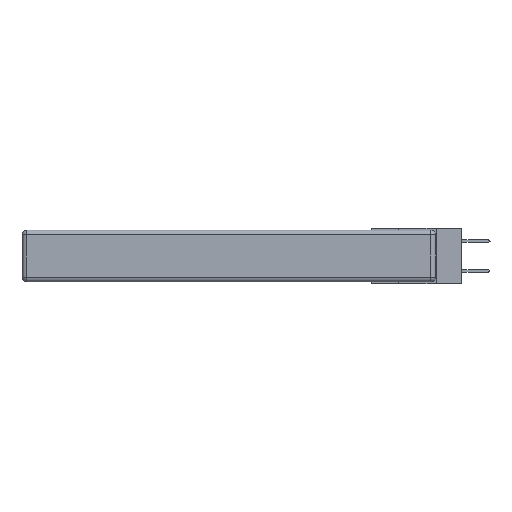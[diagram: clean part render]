
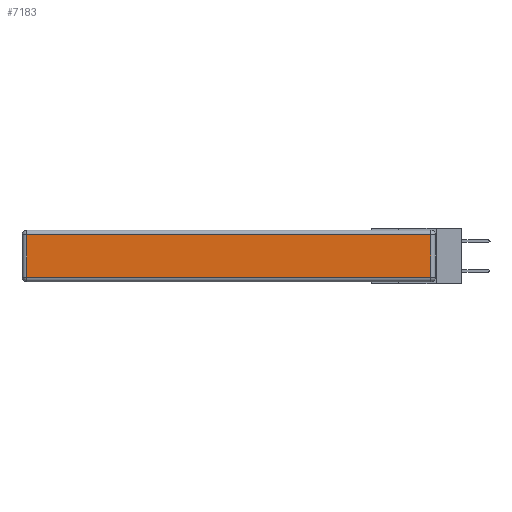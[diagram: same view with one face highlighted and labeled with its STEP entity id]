
A CAD part, left-side view. The second image highlights one B-rep face of the part: STEP entity #7183.
In plain terms, the highlighted planar face has unit normal (-1, 0, 0).
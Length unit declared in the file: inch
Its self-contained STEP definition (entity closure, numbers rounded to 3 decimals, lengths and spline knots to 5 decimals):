
#25 = ORIENTED_EDGE ( 'NONE', *, *, #5142, .T. ) ;
#563 = DIRECTION ( 'NONE',  ( 0., -1., 0. ) ) ;
#565 = CARTESIAN_POINT ( 'NONE',  ( 0., 0.03, -0.343 ) ) ;
#1200 = VECTOR ( 'NONE', #2479, 39.37008 ) ;
#1605 = DIRECTION ( 'NONE',  ( -1., 0., 0. ) ) ;
#1734 = PLANE ( 'NONE',  #2345 ) ;
#1899 = EDGE_CURVE ( 'NONE', #11422, #8645, #11143, .T. ) ;
#1921 = CARTESIAN_POINT ( 'NONE',  ( 0., 2.75, -0.03 ) ) ;
#2345 = AXIS2_PLACEMENT_3D ( 'NONE', #3602, #1605, #11135 ) ;
#2432 = CARTESIAN_POINT ( 'NONE',  ( 0., 0., -0.313 ) ) ;
#2479 = DIRECTION ( 'NONE',  ( 0., 0., 1. ) ) ;
#3174 = VECTOR ( 'NONE', #3491, 39.37008 ) ;
#3491 = DIRECTION ( 'NONE',  ( 0., 0., -1. ) ) ;
#3602 = CARTESIAN_POINT ( 'NONE',  ( 0., 0., -0.343 ) ) ;
#3911 = EDGE_LOOP ( 'NONE', ( #6838, #25, #6433, #4162 ) ) ;
#4034 = VERTEX_POINT ( 'NONE', #11706 ) ;
#4162 = ORIENTED_EDGE ( 'NONE', *, *, #7158, .T. ) ;
#5142 = EDGE_CURVE ( 'NONE', #8645, #4034, #8045, .T. ) ;
#5708 = LINE ( 'NONE', #10861, #3174 ) ;
#6433 = ORIENTED_EDGE ( 'NONE', *, *, #11928, .T. ) ;
#6634 = DIRECTION ( 'NONE',  ( 0., 1., 0. ) ) ;
#6838 = ORIENTED_EDGE ( 'NONE', *, *, #1899, .T. ) ;
#6851 = CARTESIAN_POINT ( 'NONE',  ( 0., 0.03, -0.313 ) ) ;
#7016 = VECTOR ( 'NONE', #6634, 39.37008 ) ;
#7158 = EDGE_CURVE ( 'NONE', #10282, #11422, #5708, .T. ) ;
#7183 = ADVANCED_FACE ( 'NONE', ( #7348 ), #1734, .T. ) ;
#7348 = FACE_OUTER_BOUND ( 'NONE', #3911, .T. ) ;
#8045 = LINE ( 'NONE', #565, #1200 ) ;
#8428 = CARTESIAN_POINT ( 'NONE',  ( 0., 2.72, -0.313 ) ) ;
#8590 = VECTOR ( 'NONE', #563, 39.37008 ) ;
#8645 = VERTEX_POINT ( 'NONE', #6851 ) ;
#9257 = LINE ( 'NONE', #1921, #7016 ) ;
#10029 = CARTESIAN_POINT ( 'NONE',  ( 0., 2.72, -0.03 ) ) ;
#10282 = VERTEX_POINT ( 'NONE', #10029 ) ;
#10861 = CARTESIAN_POINT ( 'NONE',  ( 0., 2.72, -0.343 ) ) ;
#11135 = DIRECTION ( 'NONE',  ( 0., 0., 1. ) ) ;
#11143 = LINE ( 'NONE', #2432, #8590 ) ;
#11422 = VERTEX_POINT ( 'NONE', #8428 ) ;
#11706 = CARTESIAN_POINT ( 'NONE',  ( 0., 0.03, -0.03 ) ) ;
#11928 = EDGE_CURVE ( 'NONE', #4034, #10282, #9257, .T. ) ;
